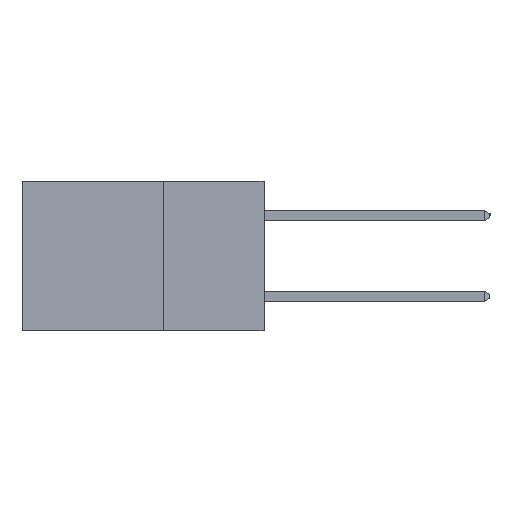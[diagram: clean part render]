
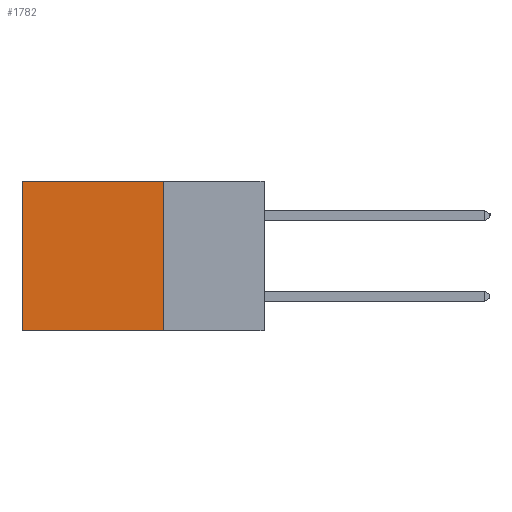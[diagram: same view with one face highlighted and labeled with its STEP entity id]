
A CAD part, left-side view. The second image highlights one B-rep face of the part: STEP entity #1782.
In plain terms, the highlighted planar face has unit normal (-1, 0, 0).
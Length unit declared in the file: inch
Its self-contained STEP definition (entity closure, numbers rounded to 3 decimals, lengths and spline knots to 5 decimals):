
#73 = VECTOR ( 'NONE', #5831, 39.37008 ) ;
#94 = CARTESIAN_POINT ( 'NONE',  ( 0.2615, 0.25, 0. ) ) ;
#745 = DIRECTION ( 'NONE',  ( 1., 0., 0. ) ) ;
#989 = CARTESIAN_POINT ( 'NONE',  ( 0.2615, 0.25, -0.37 ) ) ;
#1268 = DIRECTION ( 'NONE',  ( 0., 1., 0. ) ) ;
#1364 = EDGE_CURVE ( 'NONE', #6474, #6619, #1700, .T. ) ;
#1551 = ORIENTED_EDGE ( 'NONE', *, *, #12680, .F. ) ;
#1600 = CARTESIAN_POINT ( 'NONE',  ( 0.2615, 0.25, -0.37 ) ) ;
#1700 = LINE ( 'NONE', #7811, #1744 ) ;
#1744 = VECTOR ( 'NONE', #1268, 39.37008 ) ;
#1782 = ADVANCED_FACE ( 'NONE', ( #7139 ), #1834, .F. ) ;
#1834 = PLANE ( 'NONE',  #11828 ) ;
#2746 = EDGE_CURVE ( 'NONE', #12326, #6619, #13633, .T. ) ;
#3122 = LINE ( 'NONE', #4204, #7538 ) ;
#3193 = DIRECTION ( 'NONE',  ( 0., 0., -1. ) ) ;
#3209 = ORIENTED_EDGE ( 'NONE', *, *, #1364, .F. ) ;
#4204 = CARTESIAN_POINT ( 'NONE',  ( 0.2615, 0.25, -0.37 ) ) ;
#5162 = ORIENTED_EDGE ( 'NONE', *, *, #12801, .T. ) ;
#5686 = CARTESIAN_POINT ( 'NONE',  ( 0.2615, 0.6, -0.37 ) ) ;
#5831 = DIRECTION ( 'NONE',  ( 0., 0., -1. ) ) ;
#6042 = DIRECTION ( 'NONE',  ( 0., 0., -1. ) ) ;
#6474 = VERTEX_POINT ( 'NONE', #989 ) ;
#6619 = VERTEX_POINT ( 'NONE', #13425 ) ;
#6764 = ORIENTED_EDGE ( 'NONE', *, *, #2746, .T. ) ;
#7139 = FACE_OUTER_BOUND ( 'NONE', #11621, .T. ) ;
#7538 = VECTOR ( 'NONE', #3193, 39.37008 ) ;
#7811 = CARTESIAN_POINT ( 'NONE',  ( 0.2615, 0.25, -0.37 ) ) ;
#7872 = LINE ( 'NONE', #94, #12878 ) ;
#8841 = CARTESIAN_POINT ( 'NONE',  ( 0.2615, 0.6, 0. ) ) ;
#9932 = CARTESIAN_POINT ( 'NONE',  ( 0.2615, 0.25, 0. ) ) ;
#10745 = VERTEX_POINT ( 'NONE', #9932 ) ;
#11621 = EDGE_LOOP ( 'NONE', ( #6764, #3209, #1551, #5162 ) ) ;
#11828 = AXIS2_PLACEMENT_3D ( 'NONE', #1600, #745, #6042 ) ;
#12326 = VERTEX_POINT ( 'NONE', #8841 ) ;
#12680 = EDGE_CURVE ( 'NONE', #10745, #6474, #3122, .T. ) ;
#12801 = EDGE_CURVE ( 'NONE', #10745, #12326, #7872, .T. ) ;
#12878 = VECTOR ( 'NONE', #13415, 39.37008 ) ;
#13415 = DIRECTION ( 'NONE',  ( 0., 1., 0. ) ) ;
#13425 = CARTESIAN_POINT ( 'NONE',  ( 0.2615, 0.6, -0.37 ) ) ;
#13633 = LINE ( 'NONE', #5686, #73 ) ;
